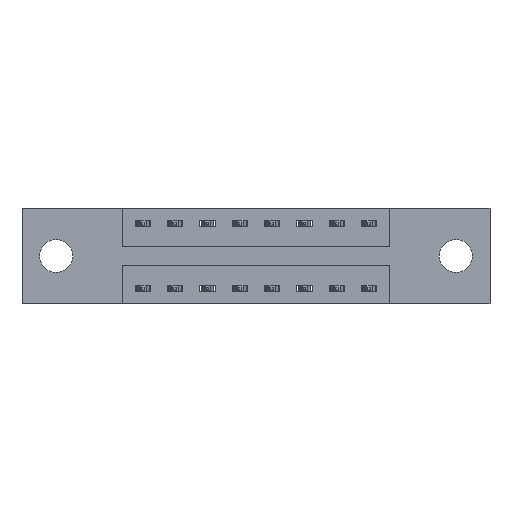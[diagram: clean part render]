
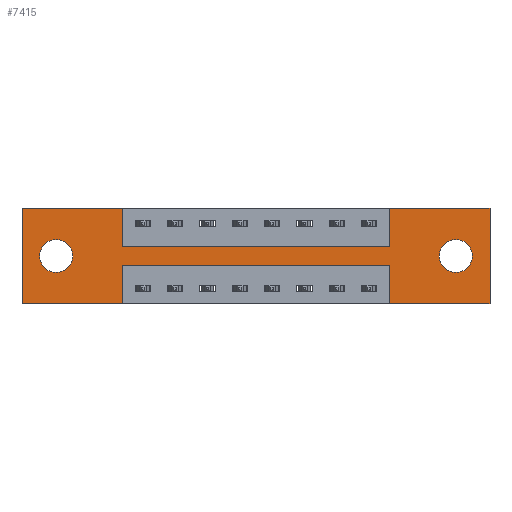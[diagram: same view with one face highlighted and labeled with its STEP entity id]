
A CAD part, front view. The second image highlights one B-rep face of the part: STEP entity #7415.
In plain terms, the highlighted planar face has unit normal (0, -1, 0).
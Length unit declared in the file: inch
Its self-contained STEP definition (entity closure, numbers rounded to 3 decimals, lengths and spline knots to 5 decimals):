
#360 = CIRCLE ( 'NONE', #6901, 0.064 ) ;
#399 = EDGE_CURVE ( 'NONE', #7090, #3856, #1046, .T. ) ;
#637 = VERTEX_POINT ( 'NONE', #7288 ) ;
#669 = ORIENTED_EDGE ( 'NONE', *, *, #9727, .F. ) ;
#793 = EDGE_CURVE ( 'NONE', #637, #2090, #814, .T. ) ;
#814 = LINE ( 'NONE', #3820, #7794 ) ;
#844 = CARTESIAN_POINT ( 'NONE',  ( 0., 0., 0. ) ) ;
#1046 = LINE ( 'NONE', #4533, #7685 ) ;
#1343 = CARTESIAN_POINT ( 'NONE',  ( 1.4225, 0., 0. ) ) ;
#1445 = CARTESIAN_POINT ( 'NONE',  ( 0.3875, 0., -0.15 ) ) ;
#1452 = VERTEX_POINT ( 'NONE', #1910 ) ;
#1486 = CARTESIAN_POINT ( 'NONE',  ( 0.1325, 0., -0.185 ) ) ;
#1502 = DIRECTION ( 'NONE',  ( 0., 0., -1. ) ) ;
#1552 = VERTEX_POINT ( 'NONE', #5124 ) ;
#1613 = CARTESIAN_POINT ( 'NONE',  ( 1.6775, 0., -0.185 ) ) ;
#1708 = DIRECTION ( 'NONE',  ( 0., 1., 0. ) ) ;
#1910 = CARTESIAN_POINT ( 'NONE',  ( 1.81, 0., -0.37 ) ) ;
#1939 = ORIENTED_EDGE ( 'NONE', *, *, #6041, .T. ) ;
#2013 = EDGE_CURVE ( 'NONE', #1452, #2814, #3641, .T. ) ;
#2083 = LINE ( 'NONE', #7079, #6647 ) ;
#2090 = VERTEX_POINT ( 'NONE', #7834 ) ;
#2184 = ORIENTED_EDGE ( 'NONE', *, *, #7265, .F. ) ;
#2197 = VECTOR ( 'NONE', #4666, 39.37008 ) ;
#2328 = LINE ( 'NONE', #9002, #9130 ) ;
#2405 = VERTEX_POINT ( 'NONE', #1445 ) ;
#2526 = DIRECTION ( 'NONE',  ( 1., 0., 0. ) ) ;
#2675 = EDGE_CURVE ( 'NONE', #6014, #6499, #3502, .T. ) ;
#2761 = DIRECTION ( 'NONE',  ( 0., 1., 0. ) ) ;
#2814 = VERTEX_POINT ( 'NONE', #6623 ) ;
#2876 = CIRCLE ( 'NONE', #6193, 0.064 ) ;
#3042 = CARTESIAN_POINT ( 'NONE',  ( 0., 0., -0.37 ) ) ;
#3101 = CARTESIAN_POINT ( 'NONE',  ( 1.6775, 0., -0.249 ) ) ;
#3290 = VECTOR ( 'NONE', #7474, 39.37008 ) ;
#3398 = EDGE_CURVE ( 'NONE', #9096, #7576, #2876, .T. ) ;
#3442 = CARTESIAN_POINT ( 'NONE',  ( 0.3875, 0., 0. ) ) ;
#3475 = CARTESIAN_POINT ( 'NONE',  ( 1.6775, 0., -0.121 ) ) ;
#3502 = LINE ( 'NONE', #844, #2197 ) ;
#3530 = VECTOR ( 'NONE', #1502, 39.37008 ) ;
#3561 = DIRECTION ( 'NONE',  ( 0., -1., 0. ) ) ;
#3596 = CARTESIAN_POINT ( 'NONE',  ( 1.6775, 0., -0.185 ) ) ;
#3641 = LINE ( 'NONE', #3042, #5424 ) ;
#3645 = ORIENTED_EDGE ( 'NONE', *, *, #7516, .F. ) ;
#3670 = DIRECTION ( 'NONE',  ( 0., 0., -1. ) ) ;
#3820 = CARTESIAN_POINT ( 'NONE',  ( 0., 0., -0.37 ) ) ;
#3828 = ORIENTED_EDGE ( 'NONE', *, *, #7960, .F. ) ;
#3856 = VERTEX_POINT ( 'NONE', #6326 ) ;
#3894 = VERTEX_POINT ( 'NONE', #5621 ) ;
#3967 = EDGE_CURVE ( 'NONE', #4794, #6014, #6000, .T. ) ;
#3979 = ORIENTED_EDGE ( 'NONE', *, *, #3989, .F. ) ;
#3989 = EDGE_CURVE ( 'NONE', #2090, #4364, #7864, .T. ) ;
#4364 = VERTEX_POINT ( 'NONE', #5950 ) ;
#4413 = ORIENTED_EDGE ( 'NONE', *, *, #3398, .T. ) ;
#4533 = CARTESIAN_POINT ( 'NONE',  ( 0.3875, 0., -0.22 ) ) ;
#4543 = VECTOR ( 'NONE', #4647, 39.37008 ) ;
#4634 = CARTESIAN_POINT ( 'NONE',  ( 1.81, 0., 0. ) ) ;
#4641 = CARTESIAN_POINT ( 'NONE',  ( 0.1325, 0., -0.185 ) ) ;
#4647 = DIRECTION ( 'NONE',  ( 0., 0., 1. ) ) ;
#4666 = DIRECTION ( 'NONE',  ( 1., 0., 0. ) ) ;
#4671 = DIRECTION ( 'NONE',  ( 0., 0., 1. ) ) ;
#4762 = DIRECTION ( 'NONE',  ( 0., 0., 1. ) ) ;
#4794 = VERTEX_POINT ( 'NONE', #6329 ) ;
#4856 = LINE ( 'NONE', #8891, #3290 ) ;
#4935 = VERTEX_POINT ( 'NONE', #3442 ) ;
#5124 = CARTESIAN_POINT ( 'NONE',  ( 0.1325, 0., -0.121 ) ) ;
#5166 = CARTESIAN_POINT ( 'NONE',  ( 0., 0., -0.37 ) ) ;
#5272 = ORIENTED_EDGE ( 'NONE', *, *, #793, .F. ) ;
#5299 = DIRECTION ( 'NONE',  ( -1., 0., 0. ) ) ;
#5315 = EDGE_CURVE ( 'NONE', #2814, #7090, #8774, .T. ) ;
#5424 = VECTOR ( 'NONE', #9230, 39.37008 ) ;
#5614 = CARTESIAN_POINT ( 'NONE',  ( 0.3875, 0., -0.15 ) ) ;
#5621 = CARTESIAN_POINT ( 'NONE',  ( 0.1325, 0., -0.249 ) ) ;
#5625 = DIRECTION ( 'NONE',  ( 0., 0., -1. ) ) ;
#5759 = EDGE_CURVE ( 'NONE', #1552, #3894, #360, .T. ) ;
#5870 = VECTOR ( 'NONE', #9820, 39.37008 ) ;
#5950 = CARTESIAN_POINT ( 'NONE',  ( 0., 0., 0. ) ) ;
#6000 = LINE ( 'NONE', #7756, #7740 ) ;
#6014 = VERTEX_POINT ( 'NONE', #1343 ) ;
#6019 = DIRECTION ( 'NONE',  ( 0., 1., 0. ) ) ;
#6041 = EDGE_CURVE ( 'NONE', #3894, #1552, #6679, .T. ) ;
#6094 = ORIENTED_EDGE ( 'NONE', *, *, #7593, .F. ) ;
#6193 = AXIS2_PLACEMENT_3D ( 'NONE', #1613, #1708, #9324 ) ;
#6251 = CARTESIAN_POINT ( 'NONE',  ( 1.81, 0., 0. ) ) ;
#6279 = LINE ( 'NONE', #5614, #6992 ) ;
#6326 = CARTESIAN_POINT ( 'NONE',  ( 0.3875, 0., -0.22 ) ) ;
#6329 = CARTESIAN_POINT ( 'NONE',  ( 1.4225, 0., -0.15 ) ) ;
#6464 = ORIENTED_EDGE ( 'NONE', *, *, #5315, .F. ) ;
#6499 = VERTEX_POINT ( 'NONE', #6251 ) ;
#6623 = CARTESIAN_POINT ( 'NONE',  ( 1.4225, 0., -0.37 ) ) ;
#6647 = VECTOR ( 'NONE', #5625, 39.37008 ) ;
#6651 = FACE_BOUND ( 'NONE', #9156, .T. ) ;
#6679 = CIRCLE ( 'NONE', #8404, 0.064 ) ;
#6744 = ORIENTED_EDGE ( 'NONE', *, *, #2675, .F. ) ;
#6807 = CARTESIAN_POINT ( 'NONE',  ( 1.4225, 0., -0.22 ) ) ;
#6901 = AXIS2_PLACEMENT_3D ( 'NONE', #4641, #7665, #4671 ) ;
#6992 = VECTOR ( 'NONE', #2526, 39.37008 ) ;
#7079 = CARTESIAN_POINT ( 'NONE',  ( 0.3875, 0., 0. ) ) ;
#7090 = VERTEX_POINT ( 'NONE', #6807 ) ;
#7147 = EDGE_CURVE ( 'NONE', #7576, #9096, #9009, .T. ) ;
#7265 = EDGE_CURVE ( 'NONE', #4364, #4935, #2328, .T. ) ;
#7288 = CARTESIAN_POINT ( 'NONE',  ( 0.3875, 0., -0.37 ) ) ;
#7415 = ADVANCED_FACE ( 'NONE', ( #9602, #6651, #8153 ), #8229, .T. ) ;
#7474 = DIRECTION ( 'NONE',  ( 0., 0., -1. ) ) ;
#7516 = EDGE_CURVE ( 'NONE', #6499, #1452, #7791, .T. ) ;
#7525 = AXIS2_PLACEMENT_3D ( 'NONE', #3596, #2761, #8892 ) ;
#7543 = ORIENTED_EDGE ( 'NONE', *, *, #2013, .F. ) ;
#7576 = VERTEX_POINT ( 'NONE', #3101 ) ;
#7593 = EDGE_CURVE ( 'NONE', #2405, #4794, #6279, .T. ) ;
#7665 = DIRECTION ( 'NONE',  ( 0., 1., 0. ) ) ;
#7685 = VECTOR ( 'NONE', #5299, 39.37008 ) ;
#7740 = VECTOR ( 'NONE', #4762, 39.37008 ) ;
#7756 = CARTESIAN_POINT ( 'NONE',  ( 1.4225, 0., 0. ) ) ;
#7791 = LINE ( 'NONE', #4634, #3530 ) ;
#7794 = VECTOR ( 'NONE', #9126, 39.37008 ) ;
#7797 = ORIENTED_EDGE ( 'NONE', *, *, #3967, .F. ) ;
#7834 = CARTESIAN_POINT ( 'NONE',  ( 0., 0., -0.37 ) ) ;
#7864 = LINE ( 'NONE', #9017, #5870 ) ;
#7960 = EDGE_CURVE ( 'NONE', #4935, #2405, #2083, .T. ) ;
#8153 = FACE_OUTER_BOUND ( 'NONE', #9527, .T. ) ;
#8203 = CARTESIAN_POINT ( 'NONE',  ( 1.4225, 0., -0.37 ) ) ;
#8229 = PLANE ( 'NONE',  #9195 ) ;
#8232 = ORIENTED_EDGE ( 'NONE', *, *, #7147, .T. ) ;
#8326 = EDGE_LOOP ( 'NONE', ( #4413, #8232 ) ) ;
#8329 = DIRECTION ( 'NONE',  ( 1., 0., 0. ) ) ;
#8404 = AXIS2_PLACEMENT_3D ( 'NONE', #1486, #6019, #8976 ) ;
#8464 = ORIENTED_EDGE ( 'NONE', *, *, #399, .F. ) ;
#8774 = LINE ( 'NONE', #8203, #4543 ) ;
#8891 = CARTESIAN_POINT ( 'NONE',  ( 0.3875, 0., -0.37 ) ) ;
#8892 = DIRECTION ( 'NONE',  ( 0., 0., -1. ) ) ;
#8976 = DIRECTION ( 'NONE',  ( 0., 0., 1. ) ) ;
#9002 = CARTESIAN_POINT ( 'NONE',  ( 0., 0., 0. ) ) ;
#9009 = CIRCLE ( 'NONE', #7525, 0.064 ) ;
#9017 = CARTESIAN_POINT ( 'NONE',  ( 0., 0., 0. ) ) ;
#9096 = VERTEX_POINT ( 'NONE', #3475 ) ;
#9126 = DIRECTION ( 'NONE',  ( -1., 0., 0. ) ) ;
#9130 = VECTOR ( 'NONE', #8329, 39.37008 ) ;
#9156 = EDGE_LOOP ( 'NONE', ( #9556, #1939 ) ) ;
#9195 = AXIS2_PLACEMENT_3D ( 'NONE', #5166, #3561, #3670 ) ;
#9230 = DIRECTION ( 'NONE',  ( -1., 0., 0. ) ) ;
#9324 = DIRECTION ( 'NONE',  ( 0., 0., -1. ) ) ;
#9527 = EDGE_LOOP ( 'NONE', ( #669, #8464, #6464, #7543, #3645, #6744, #7797, #6094, #3828, #2184, #3979, #5272 ) ) ;
#9556 = ORIENTED_EDGE ( 'NONE', *, *, #5759, .T. ) ;
#9602 = FACE_BOUND ( 'NONE', #8326, .T. ) ;
#9727 = EDGE_CURVE ( 'NONE', #3856, #637, #4856, .T. ) ;
#9820 = DIRECTION ( 'NONE',  ( 0., 0., 1. ) ) ;
